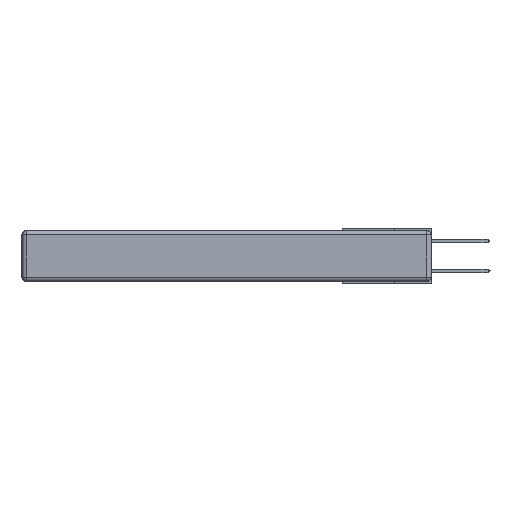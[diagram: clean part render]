
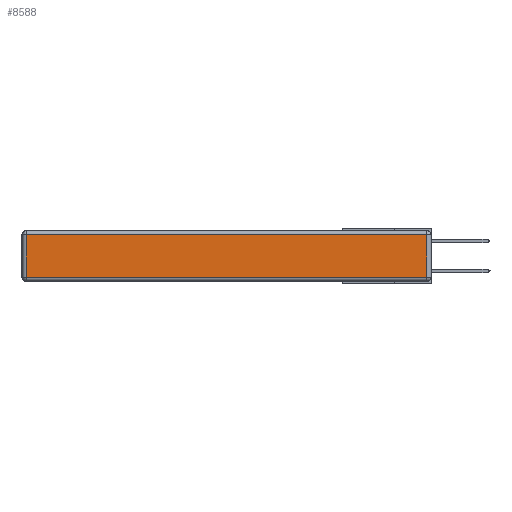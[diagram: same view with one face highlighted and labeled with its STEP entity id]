
A CAD part, left-side view. The second image highlights one B-rep face of the part: STEP entity #8588.
In plain terms, the highlighted planar face has unit normal (-1, 0, 0).
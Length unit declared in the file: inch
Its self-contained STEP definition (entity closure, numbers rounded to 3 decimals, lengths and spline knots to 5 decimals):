
#678 = CARTESIAN_POINT ( 'NONE',  ( 0., 0., -0.313 ) ) ;
#2478 = VERTEX_POINT ( 'NONE', #18696 ) ;
#2490 = ORIENTED_EDGE ( 'NONE', *, *, #12319, .T. ) ;
#2606 = LINE ( 'NONE', #15691, #19675 ) ;
#3528 = AXIS2_PLACEMENT_3D ( 'NONE', #5569, #5494, #8579 ) ;
#4316 = VECTOR ( 'NONE', #13834, 39.37008 ) ;
#4488 = LINE ( 'NONE', #10482, #17012 ) ;
#5324 = ORIENTED_EDGE ( 'NONE', *, *, #7946, .T. ) ;
#5494 = DIRECTION ( 'NONE',  ( -1., 0., 0. ) ) ;
#5569 = CARTESIAN_POINT ( 'NONE',  ( 0., 0., -0.343 ) ) ;
#6618 = ORIENTED_EDGE ( 'NONE', *, *, #10267, .T. ) ;
#6710 = CARTESIAN_POINT ( 'NONE',  ( 0., 2.72, -0.343 ) ) ;
#7321 = VERTEX_POINT ( 'NONE', #20407 ) ;
#7912 = LINE ( 'NONE', #678, #4316 ) ;
#7946 = EDGE_CURVE ( 'NONE', #10488, #2478, #4488, .T. ) ;
#8136 = DIRECTION ( 'NONE',  ( 0., 0., -1. ) ) ;
#8579 = DIRECTION ( 'NONE',  ( 0., 0., 1. ) ) ;
#8588 = ADVANCED_FACE ( 'NONE', ( #17506 ), #18527, .T. ) ;
#8841 = DIRECTION ( 'NONE',  ( 0., 1., 0. ) ) ;
#8918 = DIRECTION ( 'NONE',  ( 0., 0., 1. ) ) ;
#9017 = VECTOR ( 'NONE', #8136, 39.37008 ) ;
#10267 = EDGE_CURVE ( 'NONE', #19762, #7321, #14610, .T. ) ;
#10482 = CARTESIAN_POINT ( 'NONE',  ( 0., 0.03, -0.343 ) ) ;
#10488 = VERTEX_POINT ( 'NONE', #15261 ) ;
#10588 = EDGE_CURVE ( 'NONE', #2478, #19762, #2606, .T. ) ;
#12319 = EDGE_CURVE ( 'NONE', #7321, #10488, #7912, .T. ) ;
#13834 = DIRECTION ( 'NONE',  ( 0., -1., 0. ) ) ;
#14610 = LINE ( 'NONE', #6710, #9017 ) ;
#14642 = ORIENTED_EDGE ( 'NONE', *, *, #10588, .T. ) ;
#15261 = CARTESIAN_POINT ( 'NONE',  ( 0., 0.03, -0.313 ) ) ;
#15691 = CARTESIAN_POINT ( 'NONE',  ( 0., 2.75, -0.03 ) ) ;
#17012 = VECTOR ( 'NONE', #8918, 39.37008 ) ;
#17506 = FACE_OUTER_BOUND ( 'NONE', #18304, .T. ) ;
#18304 = EDGE_LOOP ( 'NONE', ( #2490, #5324, #14642, #6618 ) ) ;
#18527 = PLANE ( 'NONE',  #3528 ) ;
#18696 = CARTESIAN_POINT ( 'NONE',  ( 0., 0.03, -0.03 ) ) ;
#19675 = VECTOR ( 'NONE', #8841, 39.37008 ) ;
#19762 = VERTEX_POINT ( 'NONE', #20070 ) ;
#20070 = CARTESIAN_POINT ( 'NONE',  ( 0., 2.72, -0.03 ) ) ;
#20407 = CARTESIAN_POINT ( 'NONE',  ( 0., 2.72, -0.313 ) ) ;
